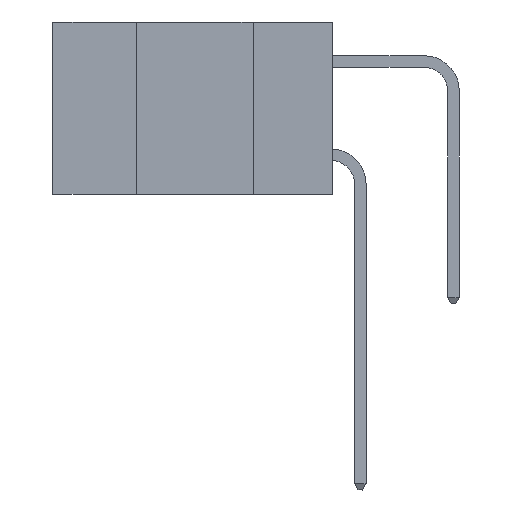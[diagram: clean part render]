
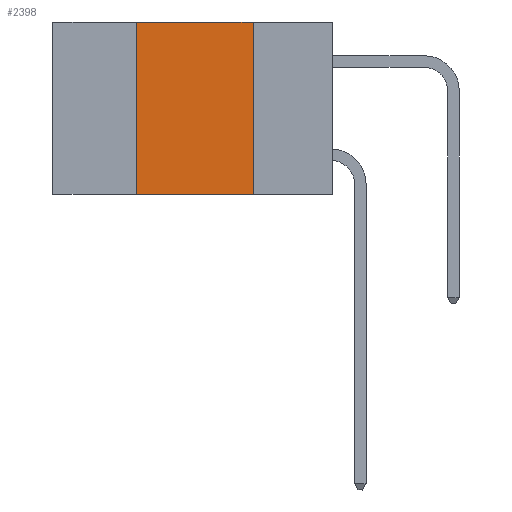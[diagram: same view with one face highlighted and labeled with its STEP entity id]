
A CAD part, left-side view. The second image highlights one B-rep face of the part: STEP entity #2398.
In plain terms, the highlighted planar face has unit normal (-1, 0, 0).
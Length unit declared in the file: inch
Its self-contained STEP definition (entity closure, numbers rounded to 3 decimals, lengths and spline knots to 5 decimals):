
#302 = VECTOR ( 'NONE', #8082, 39.37008 ) ;
#2398 = ADVANCED_FACE ( 'NONE', ( #12563 ), #11768, .F. ) ;
#2492 = VECTOR ( 'NONE', #13876, 39.37008 ) ;
#2527 = EDGE_CURVE ( 'NONE', #6206, #10066, #13541, .T. ) ;
#3703 = VERTEX_POINT ( 'NONE', #15372 ) ;
#4358 = ORIENTED_EDGE ( 'NONE', *, *, #13463, .T. ) ;
#4405 = EDGE_LOOP ( 'NONE', ( #16539, #10064, #12639, #4358 ) ) ;
#5490 = EDGE_CURVE ( 'NONE', #10066, #8250, #9568, .T. ) ;
#6206 = VERTEX_POINT ( 'NONE', #12148 ) ;
#6388 = CARTESIAN_POINT ( 'NONE',  ( 0., 0.6, -0.37 ) ) ;
#8063 = DIRECTION ( 'NONE',  ( 1., 0., 0. ) ) ;
#8082 = DIRECTION ( 'NONE',  ( 0., 0., 1. ) ) ;
#8119 = EDGE_CURVE ( 'NONE', #8250, #3703, #12161, .T. ) ;
#8246 = CARTESIAN_POINT ( 'NONE',  ( 0., 0.17, 0. ) ) ;
#8250 = VERTEX_POINT ( 'NONE', #9801 ) ;
#8547 = VECTOR ( 'NONE', #15455, 39.37008 ) ;
#8668 = VECTOR ( 'NONE', #12199, 39.37008 ) ;
#8856 = DIRECTION ( 'NONE',  ( 0., 0., -1. ) ) ;
#9568 = LINE ( 'NONE', #13053, #2492 ) ;
#9801 = CARTESIAN_POINT ( 'NONE',  ( 0., 0.17, 0. ) ) ;
#10064 = ORIENTED_EDGE ( 'NONE', *, *, #5490, .F. ) ;
#10066 = VERTEX_POINT ( 'NONE', #13573 ) ;
#10561 = CARTESIAN_POINT ( 'NONE',  ( 0., 0.42, 0. ) ) ;
#11768 = PLANE ( 'NONE',  #13295 ) ;
#12148 = CARTESIAN_POINT ( 'NONE',  ( 0., 0.42, -0.37 ) ) ;
#12161 = LINE ( 'NONE', #8246, #8668 ) ;
#12199 = DIRECTION ( 'NONE',  ( 0., 0., -1. ) ) ;
#12563 = FACE_OUTER_BOUND ( 'NONE', #4405, .T. ) ;
#12639 = ORIENTED_EDGE ( 'NONE', *, *, #2527, .F. ) ;
#13053 = CARTESIAN_POINT ( 'NONE',  ( 0., 0.6, 0. ) ) ;
#13295 = AXIS2_PLACEMENT_3D ( 'NONE', #14262, #8063, #8856 ) ;
#13463 = EDGE_CURVE ( 'NONE', #6206, #3703, #15424, .T. ) ;
#13541 = LINE ( 'NONE', #10561, #302 ) ;
#13573 = CARTESIAN_POINT ( 'NONE',  ( 0., 0.42, 0. ) ) ;
#13876 = DIRECTION ( 'NONE',  ( 0., -1., 0. ) ) ;
#14262 = CARTESIAN_POINT ( 'NONE',  ( 0., 0.6, 0. ) ) ;
#15372 = CARTESIAN_POINT ( 'NONE',  ( 0., 0.17, -0.37 ) ) ;
#15424 = LINE ( 'NONE', #6388, #8547 ) ;
#15455 = DIRECTION ( 'NONE',  ( 0., -1., 0. ) ) ;
#16539 = ORIENTED_EDGE ( 'NONE', *, *, #8119, .F. ) ;
